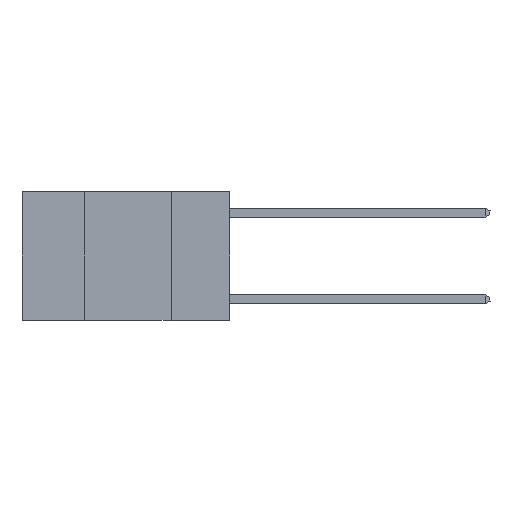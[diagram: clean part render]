
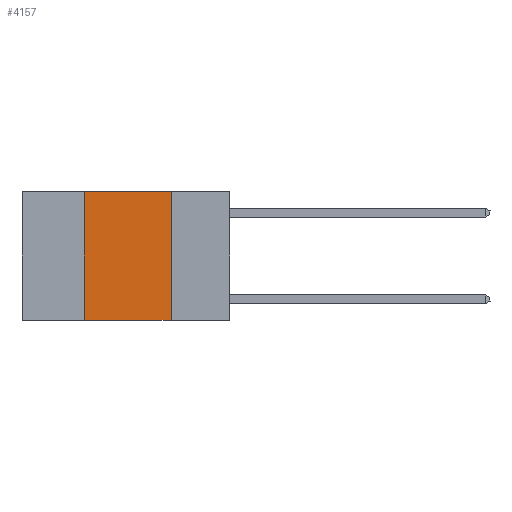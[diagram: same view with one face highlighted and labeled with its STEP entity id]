
A CAD part, left-side view. The second image highlights one B-rep face of the part: STEP entity #4157.
In plain terms, the highlighted planar face has unit normal (-1, 0, 0).
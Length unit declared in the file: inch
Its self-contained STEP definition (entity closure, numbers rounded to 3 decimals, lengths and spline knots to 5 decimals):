
#11 = VECTOR ( 'NONE', #10407, 39.37008 ) ;
#531 = LINE ( 'NONE', #5548, #11 ) ;
#902 = ORIENTED_EDGE ( 'NONE', *, *, #5210, .T. ) ;
#1320 = ORIENTED_EDGE ( 'NONE', *, *, #1889, .F. ) ;
#1597 = VECTOR ( 'NONE', #4253, 39.37008 ) ;
#1604 = EDGE_LOOP ( 'NONE', ( #1320, #19095, #4669, #902 ) ) ;
#1889 = EDGE_CURVE ( 'NONE', #5155, #16895, #15976, .T. ) ;
#2013 = CARTESIAN_POINT ( 'NONE',  ( 0., 0.17, -0.37 ) ) ;
#2835 = PLANE ( 'NONE',  #16426 ) ;
#2840 = LINE ( 'NONE', #14140, #10482 ) ;
#3125 = VECTOR ( 'NONE', #17747, 39.37008 ) ;
#3422 = FACE_OUTER_BOUND ( 'NONE', #1604, .T. ) ;
#3879 = VERTEX_POINT ( 'NONE', #5607 ) ;
#4157 = ADVANCED_FACE ( 'NONE', ( #3422 ), #2835, .F. ) ;
#4253 = DIRECTION ( 'NONE',  ( 0., -1., 0. ) ) ;
#4669 = ORIENTED_EDGE ( 'NONE', *, *, #6302, .F. ) ;
#5155 = VERTEX_POINT ( 'NONE', #18484 ) ;
#5210 = EDGE_CURVE ( 'NONE', #3879, #16895, #18731, .T. ) ;
#5548 = CARTESIAN_POINT ( 'NONE',  ( 0., 0.6, 0. ) ) ;
#5607 = CARTESIAN_POINT ( 'NONE',  ( 0., 0.42, -0.37 ) ) ;
#6156 = CARTESIAN_POINT ( 'NONE',  ( 0., 0.6, 0. ) ) ;
#6302 = EDGE_CURVE ( 'NONE', #3879, #18572, #2840, .T. ) ;
#10407 = DIRECTION ( 'NONE',  ( 0., -1., 0. ) ) ;
#10482 = VECTOR ( 'NONE', #20440, 39.37008 ) ;
#11003 = DIRECTION ( 'NONE',  ( 0., 0., -1. ) ) ;
#11150 = EDGE_CURVE ( 'NONE', #18572, #5155, #531, .T. ) ;
#13556 = CARTESIAN_POINT ( 'NONE',  ( 0., 0.42, 0. ) ) ;
#14140 = CARTESIAN_POINT ( 'NONE',  ( 0., 0.42, 0. ) ) ;
#15976 = LINE ( 'NONE', #16795, #3125 ) ;
#16426 = AXIS2_PLACEMENT_3D ( 'NONE', #6156, #20500, #11003 ) ;
#16795 = CARTESIAN_POINT ( 'NONE',  ( 0., 0.17, 0. ) ) ;
#16895 = VERTEX_POINT ( 'NONE', #2013 ) ;
#17747 = DIRECTION ( 'NONE',  ( 0., 0., -1. ) ) ;
#18484 = CARTESIAN_POINT ( 'NONE',  ( 0., 0.17, 0. ) ) ;
#18572 = VERTEX_POINT ( 'NONE', #13556 ) ;
#18731 = LINE ( 'NONE', #20196, #1597 ) ;
#19095 = ORIENTED_EDGE ( 'NONE', *, *, #11150, .F. ) ;
#20196 = CARTESIAN_POINT ( 'NONE',  ( 0., 0.6, -0.37 ) ) ;
#20440 = DIRECTION ( 'NONE',  ( 0., 0., 1. ) ) ;
#20500 = DIRECTION ( 'NONE',  ( 1., 0., 0. ) ) ;
